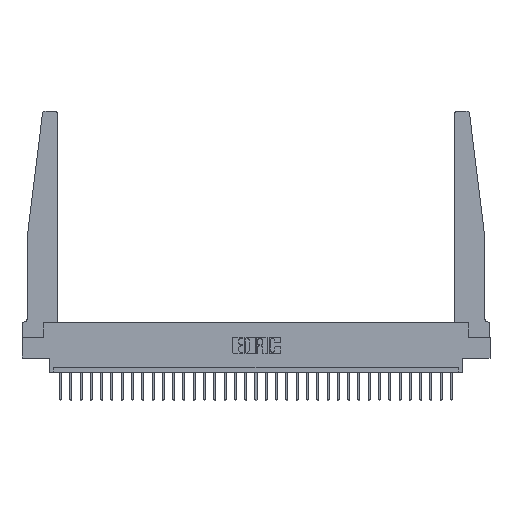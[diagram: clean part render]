
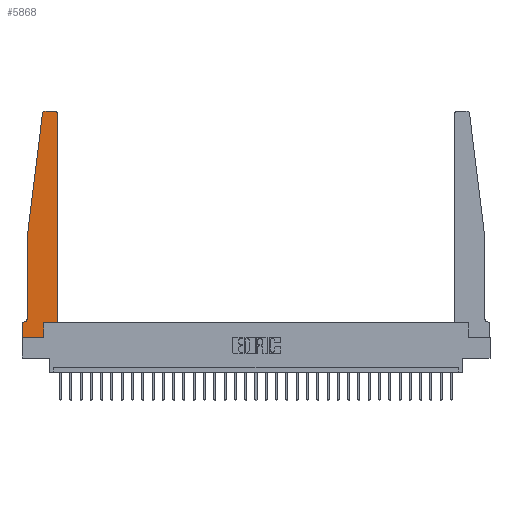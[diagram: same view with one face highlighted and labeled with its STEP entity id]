
A CAD part, top view. The second image highlights one B-rep face of the part: STEP entity #5868.
In plain terms, the highlighted planar face has unit normal (0, 0, 1).
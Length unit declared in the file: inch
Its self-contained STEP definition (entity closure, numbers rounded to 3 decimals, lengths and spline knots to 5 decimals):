
#526 = EDGE_CURVE ( 'NONE', #22764, #10108, #25122, .T. ) ;
#731 = CARTESIAN_POINT ( 'NONE',  ( 0.015, 0.1875, 0.37 ) ) ;
#1112 = VECTOR ( 'NONE', #14084, 39.37008 ) ;
#1149 = CARTESIAN_POINT ( 'NONE',  ( 0., 0.1875, 0.37 ) ) ;
#1476 = CARTESIAN_POINT ( 'NONE',  ( 0.425, 2.72, 0.37 ) ) ;
#1557 = LINE ( 'NONE', #6130, #26486 ) ;
#1601 = VERTEX_POINT ( 'NONE', #1476 ) ;
#1605 = CARTESIAN_POINT ( 'NONE',  ( 0.425, 0.18, 0.37 ) ) ;
#1856 = EDGE_CURVE ( 'NONE', #10108, #14867, #8505, .T. ) ;
#2511 = CARTESIAN_POINT ( 'NONE',  ( 0.065, 0.1875, 0.37 ) ) ;
#2752 = ORIENTED_EDGE ( 'NONE', *, *, #29211, .T. ) ;
#3031 = CARTESIAN_POINT ( 'NONE',  ( 0.395, 2.72, 0.37 ) ) ;
#3319 = CARTESIAN_POINT ( 'NONE',  ( 0.065, 1.25, 0.37 ) ) ;
#3761 = DIRECTION ( 'NONE',  ( 0., -1., 0. ) ) ;
#3861 = ORIENTED_EDGE ( 'NONE', *, *, #22635, .T. ) ;
#3937 = CARTESIAN_POINT ( 'NONE',  ( 0.24675, 2.72367, 0.37 ) ) ;
#4224 = DIRECTION ( 'NONE',  ( 0., 0., 1. ) ) ;
#4255 = ORIENTED_EDGE ( 'NONE', *, *, #526, .T. ) ;
#4922 = VERTEX_POINT ( 'NONE', #22952 ) ;
#5812 = EDGE_CURVE ( 'NONE', #20411, #14825, #27860, .T. ) ;
#5868 = ADVANCED_FACE ( 'NONE', ( #28606 ), #21947, .T. ) ;
#6130 = CARTESIAN_POINT ( 'NONE',  ( 0.2605, 0.18, 0.37 ) ) ;
#6407 = ORIENTED_EDGE ( 'NONE', *, *, #28392, .T. ) ;
#6541 = CIRCLE ( 'NONE', #11384, 0.03 ) ;
#6971 = CARTESIAN_POINT ( 'NONE',  ( 0.425, 0.18, 0.37 ) ) ;
#7098 = CARTESIAN_POINT ( 'NONE',  ( 0.065, 1.25, 0.37 ) ) ;
#7237 = CARTESIAN_POINT ( 'NONE',  ( 0.065, 0.2375, 0.37 ) ) ;
#7735 = AXIS2_PLACEMENT_3D ( 'NONE', #1149, #21806, #19225 ) ;
#8115 = VECTOR ( 'NONE', #3761, 39.37008 ) ;
#8419 = EDGE_CURVE ( 'NONE', #14867, #12439, #1557, .T. ) ;
#8505 = LINE ( 'NONE', #24124, #11102 ) ;
#8847 = DIRECTION ( 'NONE',  ( -1., 0., 0. ) ) ;
#9094 = CARTESIAN_POINT ( 'NONE',  ( 0.27653, 2.72, 0.37 ) ) ;
#9318 = VECTOR ( 'NONE', #18756, 39.37008 ) ;
#9863 = EDGE_CURVE ( 'NONE', #29857, #22764, #21019, .T. ) ;
#10108 = VERTEX_POINT ( 'NONE', #10809 ) ;
#10109 = VERTEX_POINT ( 'NONE', #14498 ) ;
#10403 = CIRCLE ( 'NONE', #27313, 0.03 ) ;
#10809 = CARTESIAN_POINT ( 'NONE',  ( 0., 0., 0.37 ) ) ;
#10892 = DIRECTION ( 'NONE',  ( 0., 1., 0. ) ) ;
#10923 = DIRECTION ( 'NONE',  ( 1., 0., 0. ) ) ;
#11102 = VECTOR ( 'NONE', #24569, 39.37008 ) ;
#11384 = AXIS2_PLACEMENT_3D ( 'NONE', #9094, #4224, #10923 ) ;
#11831 = EDGE_CURVE ( 'NONE', #1601, #10109, #10403, .T. ) ;
#12039 = CARTESIAN_POINT ( 'NONE',  ( 0.065, 1.25, 0.37 ) ) ;
#12283 = DIRECTION ( 'NONE',  ( 1., 0., 0. ) ) ;
#12296 = ORIENTED_EDGE ( 'NONE', *, *, #5812, .T. ) ;
#12393 = CARTESIAN_POINT ( 'NONE',  ( 0.25, 2.75, 0.37 ) ) ;
#12439 = VERTEX_POINT ( 'NONE', #21290 ) ;
#12834 = LINE ( 'NONE', #1605, #28976 ) ;
#13553 = EDGE_CURVE ( 'NONE', #26675, #1601, #12834, .T. ) ;
#13901 = ORIENTED_EDGE ( 'NONE', *, *, #1856, .T. ) ;
#14084 = DIRECTION ( 'NONE',  ( 1., 0., 0. ) ) ;
#14100 = ORIENTED_EDGE ( 'NONE', *, *, #11831, .T. ) ;
#14498 = CARTESIAN_POINT ( 'NONE',  ( 0.395, 2.75, 0.37 ) ) ;
#14825 = VERTEX_POINT ( 'NONE', #7237 ) ;
#14867 = VERTEX_POINT ( 'NONE', #27683 ) ;
#15264 = DIRECTION ( 'NONE',  ( -1., 0., 0. ) ) ;
#15934 = VECTOR ( 'NONE', #16357, 39.37008 ) ;
#16357 = DIRECTION ( 'NONE',  ( 0., -1., 0. ) ) ;
#16901 = VERTEX_POINT ( 'NONE', #3937 ) ;
#17147 = CIRCLE ( 'NONE', #17622, 0.05 ) ;
#17622 = AXIS2_PLACEMENT_3D ( 'NONE', #24911, #27179, #8847 ) ;
#18421 = ORIENTED_EDGE ( 'NONE', *, *, #13553, .T. ) ;
#18756 = DIRECTION ( 'NONE',  ( -1., 0., 0. ) ) ;
#18766 = EDGE_LOOP ( 'NONE', ( #26697, #27975, #3861, #12296, #2752, #20903, #4255, #13901, #20555, #6407, #18421, #14100 ) ) ;
#18814 = LINE ( 'NONE', #6971, #1112 ) ;
#18892 = CARTESIAN_POINT ( 'NONE',  ( 0., 0.1875, 0.37 ) ) ;
#19225 = DIRECTION ( 'NONE',  ( 1., 0., 0. ) ) ;
#19406 = VECTOR ( 'NONE', #15264, 39.37008 ) ;
#20411 = VERTEX_POINT ( 'NONE', #12039 ) ;
#20555 = ORIENTED_EDGE ( 'NONE', *, *, #8419, .T. ) ;
#20903 = ORIENTED_EDGE ( 'NONE', *, *, #9863, .T. ) ;
#21019 = LINE ( 'NONE', #2511, #9318 ) ;
#21290 = CARTESIAN_POINT ( 'NONE',  ( 0.2605, 0.18, 0.37 ) ) ;
#21655 = LINE ( 'NONE', #12393, #19406 ) ;
#21806 = DIRECTION ( 'NONE',  ( 0., 0., 1. ) ) ;
#21947 = PLANE ( 'NONE',  #7735 ) ;
#22130 = LINE ( 'NONE', #3319, #24154 ) ;
#22359 = DIRECTION ( 'NONE',  ( 0., 1., 0. ) ) ;
#22635 = EDGE_CURVE ( 'NONE', #16901, #20411, #22130, .T. ) ;
#22764 = VERTEX_POINT ( 'NONE', #18892 ) ;
#22896 = CARTESIAN_POINT ( 'NONE',  ( 0.425, 0.18, 0.37 ) ) ;
#22952 = CARTESIAN_POINT ( 'NONE',  ( 0.27653, 2.75, 0.37 ) ) ;
#23657 = EDGE_CURVE ( 'NONE', #4922, #16901, #6541, .T. ) ;
#23879 = EDGE_CURVE ( 'NONE', #10109, #4922, #21655, .T. ) ;
#24124 = CARTESIAN_POINT ( 'NONE',  ( 0., 0., 0.37 ) ) ;
#24154 = VECTOR ( 'NONE', #29637, 39.37008 ) ;
#24569 = DIRECTION ( 'NONE',  ( 1., 0., 0. ) ) ;
#24911 = CARTESIAN_POINT ( 'NONE',  ( 0.015, 0.2375, 0.37 ) ) ;
#25122 = LINE ( 'NONE', #29377, #8115 ) ;
#26377 = DIRECTION ( 'NONE',  ( 0., 0., 1. ) ) ;
#26486 = VECTOR ( 'NONE', #22359, 39.37008 ) ;
#26675 = VERTEX_POINT ( 'NONE', #22896 ) ;
#26697 = ORIENTED_EDGE ( 'NONE', *, *, #23879, .T. ) ;
#27179 = DIRECTION ( 'NONE',  ( 0., 0., -1. ) ) ;
#27313 = AXIS2_PLACEMENT_3D ( 'NONE', #3031, #26377, #12283 ) ;
#27683 = CARTESIAN_POINT ( 'NONE',  ( 0.2605, 0., 0.37 ) ) ;
#27860 = LINE ( 'NONE', #7098, #15934 ) ;
#27975 = ORIENTED_EDGE ( 'NONE', *, *, #23657, .T. ) ;
#28392 = EDGE_CURVE ( 'NONE', #12439, #26675, #18814, .T. ) ;
#28606 = FACE_OUTER_BOUND ( 'NONE', #18766, .T. ) ;
#28976 = VECTOR ( 'NONE', #10892, 39.37008 ) ;
#29211 = EDGE_CURVE ( 'NONE', #14825, #29857, #17147, .T. ) ;
#29377 = CARTESIAN_POINT ( 'NONE',  ( 0., 0., 0.37 ) ) ;
#29637 = DIRECTION ( 'NONE',  ( -0.122, -0.992, 0. ) ) ;
#29857 = VERTEX_POINT ( 'NONE', #731 ) ;
